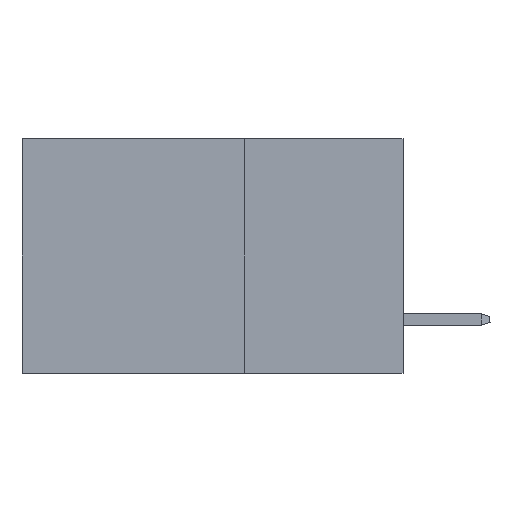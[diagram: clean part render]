
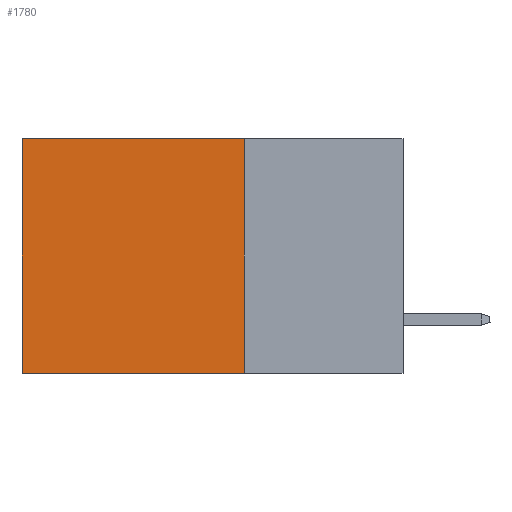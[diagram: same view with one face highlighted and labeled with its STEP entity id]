
A CAD part, left-side view. The second image highlights one B-rep face of the part: STEP entity #1780.
In plain terms, the highlighted planar face has unit normal (-1, 0, 0).
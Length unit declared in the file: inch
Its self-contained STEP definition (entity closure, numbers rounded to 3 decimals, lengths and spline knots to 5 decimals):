
#440 = CARTESIAN_POINT ( 'NONE',  ( 0.2875, 0.25, -0.37 ) ) ;
#1780 = ADVANCED_FACE ( 'NONE', ( #14050 ), #28157, .F. ) ;
#2662 = VERTEX_POINT ( 'NONE', #8670 ) ;
#3597 = DIRECTION ( 'NONE',  ( 0., 0., -1. ) ) ;
#3674 = VECTOR ( 'NONE', #18479, 39.37008 ) ;
#4419 = CARTESIAN_POINT ( 'NONE',  ( 0.2875, 0.6, -0.37 ) ) ;
#4918 = EDGE_CURVE ( 'NONE', #10019, #30191, #19153, .T. ) ;
#5468 = EDGE_CURVE ( 'NONE', #2662, #10019, #8012, .T. ) ;
#5782 = ORIENTED_EDGE ( 'NONE', *, *, #5468, .F. ) ;
#8012 = LINE ( 'NONE', #17725, #9406 ) ;
#8514 = CARTESIAN_POINT ( 'NONE',  ( 0.2875, 0.6, 0. ) ) ;
#8670 = CARTESIAN_POINT ( 'NONE',  ( 0.2875, 0.25, 0. ) ) ;
#8937 = CARTESIAN_POINT ( 'NONE',  ( 0.2875, 0.6, 0. ) ) ;
#9406 = VECTOR ( 'NONE', #26774, 39.37008 ) ;
#10019 = VERTEX_POINT ( 'NONE', #20679 ) ;
#12112 = DIRECTION ( 'NONE',  ( 0., 1., 0. ) ) ;
#14032 = VECTOR ( 'NONE', #30656, 39.37008 ) ;
#14050 = FACE_OUTER_BOUND ( 'NONE', #14477, .T. ) ;
#14110 = AXIS2_PLACEMENT_3D ( 'NONE', #23647, #15543, #3597 ) ;
#14477 = EDGE_LOOP ( 'NONE', ( #24387, #21244, #5782, #20932 ) ) ;
#15543 = DIRECTION ( 'NONE',  ( 1., 0., 0. ) ) ;
#17725 = CARTESIAN_POINT ( 'NONE',  ( 0.2875, 0.25, 0. ) ) ;
#18479 = DIRECTION ( 'NONE',  ( 0., 0., -1. ) ) ;
#19153 = LINE ( 'NONE', #440, #23398 ) ;
#19496 = VERTEX_POINT ( 'NONE', #8514 ) ;
#20679 = CARTESIAN_POINT ( 'NONE',  ( 0.2875, 0.25, -0.37 ) ) ;
#20819 = LINE ( 'NONE', #8937, #3674 ) ;
#20932 = ORIENTED_EDGE ( 'NONE', *, *, #27423, .T. ) ;
#21091 = CARTESIAN_POINT ( 'NONE',  ( 0.2875, 0.25, 0. ) ) ;
#21244 = ORIENTED_EDGE ( 'NONE', *, *, #4918, .F. ) ;
#23398 = VECTOR ( 'NONE', #12112, 39.37008 ) ;
#23647 = CARTESIAN_POINT ( 'NONE',  ( 0.2875, 0.25, 0. ) ) ;
#24387 = ORIENTED_EDGE ( 'NONE', *, *, #28262, .T. ) ;
#26774 = DIRECTION ( 'NONE',  ( 0., 0., -1. ) ) ;
#27423 = EDGE_CURVE ( 'NONE', #2662, #19496, #30193, .T. ) ;
#28157 = PLANE ( 'NONE',  #14110 ) ;
#28262 = EDGE_CURVE ( 'NONE', #19496, #30191, #20819, .T. ) ;
#30191 = VERTEX_POINT ( 'NONE', #4419 ) ;
#30193 = LINE ( 'NONE', #21091, #14032 ) ;
#30656 = DIRECTION ( 'NONE',  ( 0., 1., 0. ) ) ;
